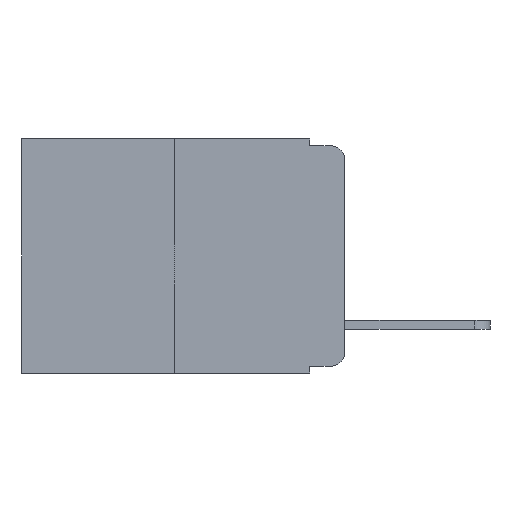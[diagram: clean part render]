
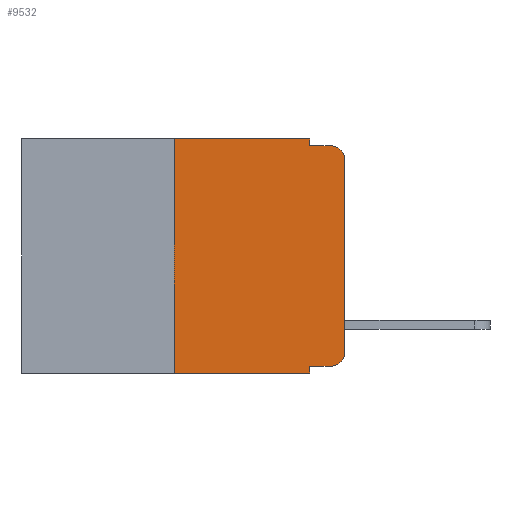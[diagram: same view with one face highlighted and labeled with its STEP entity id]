
A CAD part, left-side view. The second image highlights one B-rep face of the part: STEP entity #9532.
In plain terms, the highlighted planar face has unit normal (-1, 0, 0).
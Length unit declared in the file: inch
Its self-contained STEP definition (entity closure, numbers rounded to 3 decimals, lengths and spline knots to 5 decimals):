
#31 = ORIENTED_EDGE ( 'NONE', *, *, #5606, .T. ) ;
#281 = CARTESIAN_POINT ( 'NONE',  ( 0., 0.051, -0.333 ) ) ;
#328 = DIRECTION ( 'NONE',  ( 0., 0., -1. ) ) ;
#372 = DIRECTION ( 'NONE',  ( 1., 0., 0. ) ) ;
#414 = VERTEX_POINT ( 'NONE', #899 ) ;
#521 = CARTESIAN_POINT ( 'NONE',  ( 0., 0.473, 0. ) ) ;
#579 = DIRECTION ( 'NONE',  ( 0., -1., 0. ) ) ;
#620 = VECTOR ( 'NONE', #956, 39.37008 ) ;
#638 = LINE ( 'NONE', #792, #620 ) ;
#722 = PLANE ( 'NONE',  #5279 ) ;
#792 = CARTESIAN_POINT ( 'NONE',  ( 0., 0.051, 0. ) ) ;
#812 = VERTEX_POINT ( 'NONE', #8975 ) ;
#899 = CARTESIAN_POINT ( 'NONE',  ( 0., 0.02, -0.333 ) ) ;
#901 = VERTEX_POINT ( 'NONE', #9605 ) ;
#956 = DIRECTION ( 'NONE',  ( 0., 0., -1. ) ) ;
#1206 = EDGE_CURVE ( 'NONE', #4141, #7403, #6556, .T. ) ;
#1234 = ORIENTED_EDGE ( 'NONE', *, *, #1956, .F. ) ;
#1273 = VERTEX_POINT ( 'NONE', #6826 ) ;
#1597 = EDGE_LOOP ( 'NONE', ( #31, #6219, #6171, #1699, #10307, #1234, #10677, #9788, #9743, #5460 ) ) ;
#1699 = ORIENTED_EDGE ( 'NONE', *, *, #2542, .F. ) ;
#1745 = DIRECTION ( 'NONE',  ( 0., -1., 0. ) ) ;
#1755 = CARTESIAN_POINT ( 'NONE',  ( 0., 0., 0. ) ) ;
#1769 = CARTESIAN_POINT ( 'NONE',  ( 0., 0.473, 0. ) ) ;
#1905 = DIRECTION ( 'NONE',  ( 0., 0., 1. ) ) ;
#1942 = EDGE_CURVE ( 'NONE', #10452, #1273, #2321, .T. ) ;
#1956 = EDGE_CURVE ( 'NONE', #4141, #812, #2222, .T. ) ;
#2157 = VECTOR ( 'NONE', #8039, 39.37008 ) ;
#2202 = VECTOR ( 'NONE', #5535, 39.37008 ) ;
#2222 = LINE ( 'NONE', #5359, #2157 ) ;
#2321 = LINE ( 'NONE', #5573, #2202 ) ;
#2542 = EDGE_CURVE ( 'NONE', #901, #10452, #638, .T. ) ;
#2548 = CARTESIAN_POINT ( 'NONE',  ( 0., 0.051, -0.343 ) ) ;
#2558 = CARTESIAN_POINT ( 'NONE',  ( 0., 0.051, 0. ) ) ;
#3054 = LINE ( 'NONE', #2558, #7441 ) ;
#3123 = EDGE_CURVE ( 'NONE', #5814, #414, #5822, .T. ) ;
#3341 = VECTOR ( 'NONE', #1905, 39.37008 ) ;
#3474 = FACE_OUTER_BOUND ( 'NONE', #1597, .T. ) ;
#3806 = DIRECTION ( 'NONE',  ( 0., 0., -1. ) ) ;
#3843 = DIRECTION ( 'NONE',  ( -1., 0., 0. ) ) ;
#4141 = VERTEX_POINT ( 'NONE', #10577 ) ;
#4262 = CARTESIAN_POINT ( 'NONE',  ( 0., 0.02, -0.03 ) ) ;
#4803 = EDGE_CURVE ( 'NONE', #812, #901, #6548, .T. ) ;
#4864 = CARTESIAN_POINT ( 'NONE',  ( 0., 0., -0.03 ) ) ;
#4974 = EDGE_CURVE ( 'NONE', #5814, #7403, #3054, .T. ) ;
#5071 = AXIS2_PLACEMENT_3D ( 'NONE', #4262, #3843, #3806 ) ;
#5279 = AXIS2_PLACEMENT_3D ( 'NONE', #521, #372, #328 ) ;
#5341 = VERTEX_POINT ( 'NONE', #10231 ) ;
#5359 = CARTESIAN_POINT ( 'NONE',  ( 0., 0.25, 0. ) ) ;
#5460 = ORIENTED_EDGE ( 'NONE', *, *, #6017, .T. ) ;
#5535 = DIRECTION ( 'NONE',  ( 0., -1., 0. ) ) ;
#5573 = CARTESIAN_POINT ( 'NONE',  ( 0., 0.051, -0.01 ) ) ;
#5606 = EDGE_CURVE ( 'NONE', #5341, #6822, #9365, .T. ) ;
#5814 = VERTEX_POINT ( 'NONE', #281 ) ;
#5822 = LINE ( 'NONE', #6847, #7738 ) ;
#6017 = EDGE_CURVE ( 'NONE', #414, #5341, #9574, .T. ) ;
#6133 = VECTOR ( 'NONE', #7855, 39.37008 ) ;
#6171 = ORIENTED_EDGE ( 'NONE', *, *, #1942, .F. ) ;
#6219 = ORIENTED_EDGE ( 'NONE', *, *, #9926, .T. ) ;
#6373 = CIRCLE ( 'NONE', #5071, 0.02 ) ;
#6548 = LINE ( 'NONE', #1769, #10169 ) ;
#6556 = LINE ( 'NONE', #8601, #6133 ) ;
#6822 = VERTEX_POINT ( 'NONE', #4864 ) ;
#6826 = CARTESIAN_POINT ( 'NONE',  ( 0., 0.02, -0.01 ) ) ;
#6847 = CARTESIAN_POINT ( 'NONE',  ( 0., 0.051, -0.333 ) ) ;
#7403 = VERTEX_POINT ( 'NONE', #2548 ) ;
#7441 = VECTOR ( 'NONE', #10186, 39.37008 ) ;
#7738 = VECTOR ( 'NONE', #579, 39.37008 ) ;
#7763 = CARTESIAN_POINT ( 'NONE',  ( 0., 0.051, -0.01 ) ) ;
#7855 = DIRECTION ( 'NONE',  ( 0., -1., 0. ) ) ;
#7927 = AXIS2_PLACEMENT_3D ( 'NONE', #8336, #10440, #10689 ) ;
#8039 = DIRECTION ( 'NONE',  ( 0., 0., 1. ) ) ;
#8336 = CARTESIAN_POINT ( 'NONE',  ( 0., 0.02, -0.313 ) ) ;
#8601 = CARTESIAN_POINT ( 'NONE',  ( 0., 0.473, -0.343 ) ) ;
#8975 = CARTESIAN_POINT ( 'NONE',  ( 0., 0.25, 0. ) ) ;
#9365 = LINE ( 'NONE', #1755, #3341 ) ;
#9532 = ADVANCED_FACE ( 'NONE', ( #3474 ), #722, .F. ) ;
#9574 = CIRCLE ( 'NONE', #7927, 0.02 ) ;
#9605 = CARTESIAN_POINT ( 'NONE',  ( 0., 0.051, 0. ) ) ;
#9743 = ORIENTED_EDGE ( 'NONE', *, *, #3123, .T. ) ;
#9788 = ORIENTED_EDGE ( 'NONE', *, *, #4974, .F. ) ;
#9926 = EDGE_CURVE ( 'NONE', #6822, #1273, #6373, .T. ) ;
#10169 = VECTOR ( 'NONE', #1745, 39.37008 ) ;
#10186 = DIRECTION ( 'NONE',  ( 0., 0., -1. ) ) ;
#10231 = CARTESIAN_POINT ( 'NONE',  ( 0., 0., -0.313 ) ) ;
#10307 = ORIENTED_EDGE ( 'NONE', *, *, #4803, .F. ) ;
#10440 = DIRECTION ( 'NONE',  ( -1., 0., 0. ) ) ;
#10452 = VERTEX_POINT ( 'NONE', #7763 ) ;
#10577 = CARTESIAN_POINT ( 'NONE',  ( 0., 0.25, -0.343 ) ) ;
#10677 = ORIENTED_EDGE ( 'NONE', *, *, #1206, .T. ) ;
#10689 = DIRECTION ( 'NONE',  ( 0., 0., -1. ) ) ;
